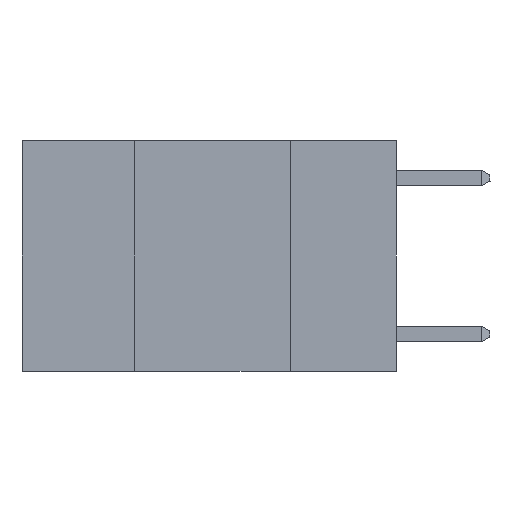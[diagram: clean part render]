
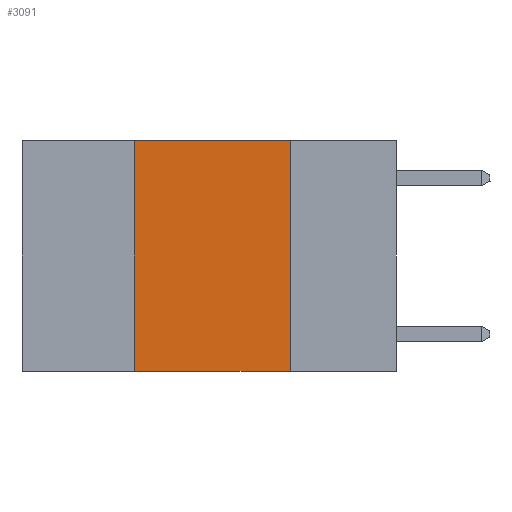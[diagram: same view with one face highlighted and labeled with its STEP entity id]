
A CAD part, left-side view. The second image highlights one B-rep face of the part: STEP entity #3091.
In plain terms, the highlighted planar face has unit normal (-1, 0, 0).
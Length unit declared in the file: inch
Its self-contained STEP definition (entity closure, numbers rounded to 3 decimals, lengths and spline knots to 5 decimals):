
#74 = CARTESIAN_POINT ( 'NONE',  ( 0., 0.6, 0. ) ) ;
#286 = CARTESIAN_POINT ( 'NONE',  ( 0., 0.17, 0. ) ) ;
#1000 = DIRECTION ( 'NONE',  ( 0., 0., -1. ) ) ;
#1899 = CARTESIAN_POINT ( 'NONE',  ( 0., 0.17, 0. ) ) ;
#1912 = LINE ( 'NONE', #1899, #5859 ) ;
#2236 = VECTOR ( 'NONE', #10345, 39.37008 ) ;
#2405 = VERTEX_POINT ( 'NONE', #3479 ) ;
#3091 = ADVANCED_FACE ( 'NONE', ( #4001 ), #5169, .F. ) ;
#3302 = LINE ( 'NONE', #8807, #5548 ) ;
#3479 = CARTESIAN_POINT ( 'NONE',  ( 0., 0.17, -0.37 ) ) ;
#4001 = FACE_OUTER_BOUND ( 'NONE', #10252, .T. ) ;
#4448 = VECTOR ( 'NONE', #5546, 39.37008 ) ;
#4502 = LINE ( 'NONE', #8820, #2236 ) ;
#4613 = ORIENTED_EDGE ( 'NONE', *, *, #8772, .F. ) ;
#4705 = LINE ( 'NONE', #4721, #4448 ) ;
#4721 = CARTESIAN_POINT ( 'NONE',  ( 0., 0.6, 0. ) ) ;
#4773 = VERTEX_POINT ( 'NONE', #5505 ) ;
#5169 = PLANE ( 'NONE',  #8540 ) ;
#5281 = DIRECTION ( 'NONE',  ( 0., 0., -1. ) ) ;
#5505 = CARTESIAN_POINT ( 'NONE',  ( 0., 0.42, -0.37 ) ) ;
#5546 = DIRECTION ( 'NONE',  ( 0., -1., 0. ) ) ;
#5548 = VECTOR ( 'NONE', #6583, 39.37008 ) ;
#5682 = EDGE_CURVE ( 'NONE', #4773, #9407, #4502, .T. ) ;
#5859 = VECTOR ( 'NONE', #5281, 39.37008 ) ;
#5997 = DIRECTION ( 'NONE',  ( 1., 0., 0. ) ) ;
#6461 = ORIENTED_EDGE ( 'NONE', *, *, #8296, .F. ) ;
#6583 = DIRECTION ( 'NONE',  ( 0., -1., 0. ) ) ;
#6687 = VERTEX_POINT ( 'NONE', #286 ) ;
#7594 = CARTESIAN_POINT ( 'NONE',  ( 0., 0.42, 0. ) ) ;
#8296 = EDGE_CURVE ( 'NONE', #9407, #6687, #4705, .T. ) ;
#8540 = AXIS2_PLACEMENT_3D ( 'NONE', #74, #5997, #1000 ) ;
#8772 = EDGE_CURVE ( 'NONE', #6687, #2405, #1912, .T. ) ;
#8807 = CARTESIAN_POINT ( 'NONE',  ( 0., 0.6, -0.37 ) ) ;
#8820 = CARTESIAN_POINT ( 'NONE',  ( 0., 0.42, 0. ) ) ;
#9265 = ORIENTED_EDGE ( 'NONE', *, *, #10079, .T. ) ;
#9280 = ORIENTED_EDGE ( 'NONE', *, *, #5682, .F. ) ;
#9407 = VERTEX_POINT ( 'NONE', #7594 ) ;
#10079 = EDGE_CURVE ( 'NONE', #4773, #2405, #3302, .T. ) ;
#10252 = EDGE_LOOP ( 'NONE', ( #4613, #6461, #9280, #9265 ) ) ;
#10345 = DIRECTION ( 'NONE',  ( 0., 0., 1. ) ) ;
